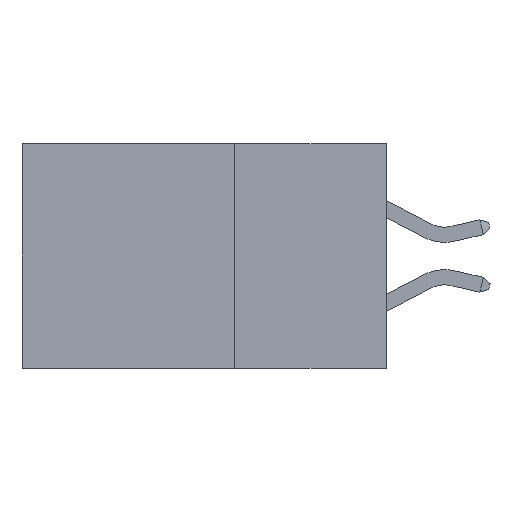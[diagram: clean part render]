
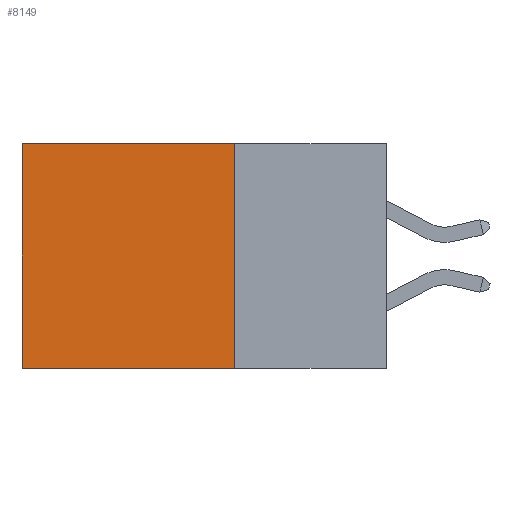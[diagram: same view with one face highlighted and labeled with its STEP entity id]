
A CAD part, left-side view. The second image highlights one B-rep face of the part: STEP entity #8149.
In plain terms, the highlighted planar face has unit normal (-1, 0, 0).
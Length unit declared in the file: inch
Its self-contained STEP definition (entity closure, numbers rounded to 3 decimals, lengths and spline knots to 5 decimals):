
#232 = CARTESIAN_POINT ( 'NONE',  ( 0.298, 0.25, -0.37 ) ) ;
#378 = LINE ( 'NONE', #5195, #8499 ) ;
#655 = VERTEX_POINT ( 'NONE', #3698 ) ;
#1197 = ORIENTED_EDGE ( 'NONE', *, *, #4079, .F. ) ;
#1232 = LINE ( 'NONE', #232, #1885 ) ;
#1789 = VERTEX_POINT ( 'NONE', #9660 ) ;
#1885 = VECTOR ( 'NONE', #2645, 39.37008 ) ;
#2645 = DIRECTION ( 'NONE',  ( 0., 1., 0. ) ) ;
#3025 = VECTOR ( 'NONE', #6642, 39.37008 ) ;
#3117 = LINE ( 'NONE', #3442, #9412 ) ;
#3155 = PLANE ( 'NONE',  #3726 ) ;
#3240 = EDGE_CURVE ( 'NONE', #9983, #655, #378, .T. ) ;
#3267 = CARTESIAN_POINT ( 'NONE',  ( 0.298, 0.6, 0. ) ) ;
#3442 = CARTESIAN_POINT ( 'NONE',  ( 0.298, 0.25, 0. ) ) ;
#3698 = CARTESIAN_POINT ( 'NONE',  ( 0.298, 0.6, 0. ) ) ;
#3726 = AXIS2_PLACEMENT_3D ( 'NONE', #10663, #10697, #8867 ) ;
#4079 = EDGE_CURVE ( 'NONE', #9983, #7783, #3117, .T. ) ;
#4969 = CARTESIAN_POINT ( 'NONE',  ( 0.298, 0.25, 0. ) ) ;
#4972 = CARTESIAN_POINT ( 'NONE',  ( 0.298, 0.25, -0.37 ) ) ;
#5180 = ORIENTED_EDGE ( 'NONE', *, *, #5931, .F. ) ;
#5195 = CARTESIAN_POINT ( 'NONE',  ( 0.298, 0.25, 0. ) ) ;
#5469 = ORIENTED_EDGE ( 'NONE', *, *, #3240, .T. ) ;
#5895 = DIRECTION ( 'NONE',  ( 0., 0., -1. ) ) ;
#5931 = EDGE_CURVE ( 'NONE', #7783, #1789, #1232, .T. ) ;
#6642 = DIRECTION ( 'NONE',  ( 0., 0., -1. ) ) ;
#7742 = FACE_OUTER_BOUND ( 'NONE', #8837, .T. ) ;
#7783 = VERTEX_POINT ( 'NONE', #4972 ) ;
#8149 = ADVANCED_FACE ( 'NONE', ( #7742 ), #3155, .F. ) ;
#8499 = VECTOR ( 'NONE', #8694, 39.37008 ) ;
#8694 = DIRECTION ( 'NONE',  ( 0., 1., 0. ) ) ;
#8789 = EDGE_CURVE ( 'NONE', #655, #1789, #10228, .T. ) ;
#8837 = EDGE_LOOP ( 'NONE', ( #9950, #5180, #1197, #5469 ) ) ;
#8867 = DIRECTION ( 'NONE',  ( 0., 0., -1. ) ) ;
#9412 = VECTOR ( 'NONE', #5895, 39.37008 ) ;
#9660 = CARTESIAN_POINT ( 'NONE',  ( 0.298, 0.6, -0.37 ) ) ;
#9950 = ORIENTED_EDGE ( 'NONE', *, *, #8789, .T. ) ;
#9983 = VERTEX_POINT ( 'NONE', #4969 ) ;
#10228 = LINE ( 'NONE', #3267, #3025 ) ;
#10663 = CARTESIAN_POINT ( 'NONE',  ( 0.298, 0.25, 0. ) ) ;
#10697 = DIRECTION ( 'NONE',  ( 1., 0., 0. ) ) ;
